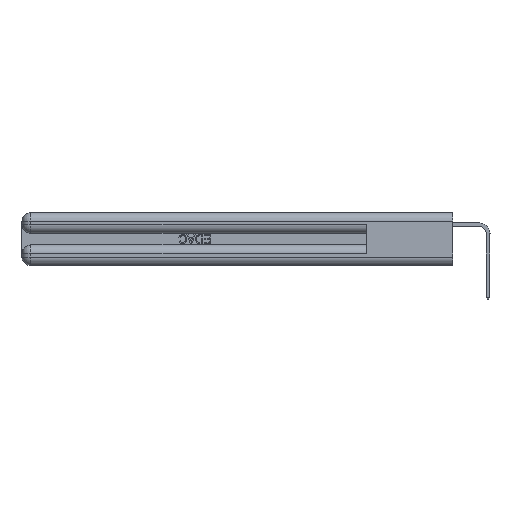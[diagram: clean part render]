
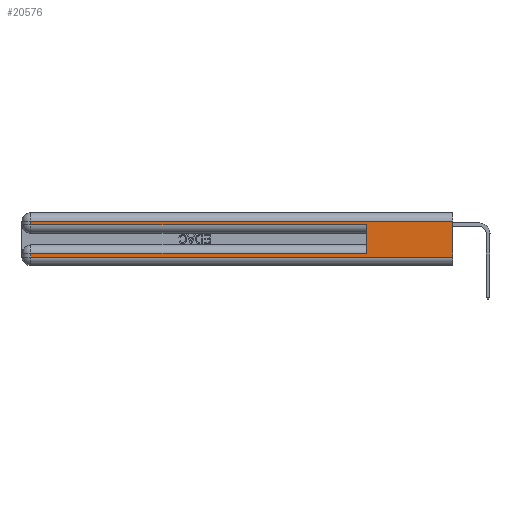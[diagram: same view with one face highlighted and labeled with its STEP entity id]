
A CAD part, left-side view. The second image highlights one B-rep face of the part: STEP entity #20576.
In plain terms, the highlighted planar face has unit normal (-1, 0, 0).
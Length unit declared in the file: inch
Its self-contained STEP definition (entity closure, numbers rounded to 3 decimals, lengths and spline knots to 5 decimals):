
#133 = ORIENTED_EDGE ( 'NONE', *, *, #24252, .T. ) ;
#1194 = DIRECTION ( 'NONE',  ( 0., 0., -1. ) ) ;
#2935 = CARTESIAN_POINT ( 'NONE',  ( 0., 0., 0.06 ) ) ;
#2998 = CARTESIAN_POINT ( 'NONE',  ( 0., 0., 0.37 ) ) ;
#3465 = VERTEX_POINT ( 'NONE', #11335 ) ;
#4004 = CARTESIAN_POINT ( 'NONE',  ( 0., 0.6, 0.085 ) ) ;
#6084 = CARTESIAN_POINT ( 'NONE',  ( 0., 0., 0.37 ) ) ;
#8313 = ORIENTED_EDGE ( 'NONE', *, *, #27761, .T. ) ;
#8512 = VECTOR ( 'NONE', #30366, 39.37008 ) ;
#9287 = VECTOR ( 'NONE', #34190, 39.37008 ) ;
#9555 = VERTEX_POINT ( 'NONE', #49953 ) ;
#9763 = LINE ( 'NONE', #2998, #8512 ) ;
#10040 = DIRECTION ( 'NONE',  ( 0., 0., -1. ) ) ;
#11335 = CARTESIAN_POINT ( 'NONE',  ( 0., 2.94, 0.085 ) ) ;
#12942 = CARTESIAN_POINT ( 'NONE',  ( 0., 2.94, 0.37 ) ) ;
#12971 = ORIENTED_EDGE ( 'NONE', *, *, #31565, .F. ) ;
#13448 = ORIENTED_EDGE ( 'NONE', *, *, #25175, .T. ) ;
#13762 = VECTOR ( 'NONE', #42012, 39.37008 ) ;
#15548 = ORIENTED_EDGE ( 'NONE', *, *, #28218, .T. ) ;
#15988 = VERTEX_POINT ( 'NONE', #4004 ) ;
#17159 = VECTOR ( 'NONE', #33457, 39.37008 ) ;
#17168 = VERTEX_POINT ( 'NONE', #26956 ) ;
#18321 = CARTESIAN_POINT ( 'NONE',  ( 0., 0.6, 0.145 ) ) ;
#20576 = ADVANCED_FACE ( 'NONE', ( #29688 ), #48687, .F. ) ;
#24252 = EDGE_CURVE ( 'NONE', #3465, #46593, #37487, .T. ) ;
#24540 = EDGE_LOOP ( 'NONE', ( #46017, #38470, #13448, #15548, #12971, #46835, #133, #8313 ) ) ;
#24818 = CARTESIAN_POINT ( 'NONE',  ( 0., 0., 0.06 ) ) ;
#24884 = VECTOR ( 'NONE', #47557, 39.37008 ) ;
#25175 = EDGE_CURVE ( 'NONE', #27025, #17168, #44715, .T. ) ;
#25419 = DIRECTION ( 'NONE',  ( 0., 1., 0. ) ) ;
#26956 = CARTESIAN_POINT ( 'NONE',  ( 0., 2.94, 0.285 ) ) ;
#27025 = VERTEX_POINT ( 'NONE', #48936 ) ;
#27183 = VECTOR ( 'NONE', #1194, 39.37008 ) ;
#27510 = LINE ( 'NONE', #44955, #17159 ) ;
#27761 = EDGE_CURVE ( 'NONE', #46593, #43760, #40271, .T. ) ;
#27945 = CARTESIAN_POINT ( 'NONE',  ( 0., 0., 0.085 ) ) ;
#28218 = EDGE_CURVE ( 'NONE', #17168, #9555, #27510, .T. ) ;
#29688 = FACE_OUTER_BOUND ( 'NONE', #24540, .T. ) ;
#30068 = CARTESIAN_POINT ( 'NONE',  ( 0., 2.94, 0.06 ) ) ;
#30366 = DIRECTION ( 'NONE',  ( 0., 0., -1. ) ) ;
#31565 = EDGE_CURVE ( 'NONE', #15988, #9555, #48326, .T. ) ;
#32401 = VERTEX_POINT ( 'NONE', #42156 ) ;
#33327 = AXIS2_PLACEMENT_3D ( 'NONE', #6084, #33336, #10040 ) ;
#33336 = DIRECTION ( 'NONE',  ( 1., 0., 0. ) ) ;
#33457 = DIRECTION ( 'NONE',  ( 0., -1., 0. ) ) ;
#34190 = DIRECTION ( 'NONE',  ( 0., -1., 0. ) ) ;
#35109 = EDGE_CURVE ( 'NONE', #32401, #43760, #9763, .T. ) ;
#36591 = VECTOR ( 'NONE', #25419, 39.37008 ) ;
#37487 = LINE ( 'NONE', #12942, #27183 ) ;
#37796 = LINE ( 'NONE', #44728, #36591 ) ;
#38128 = CARTESIAN_POINT ( 'NONE',  ( 0., 2.94, 0.37 ) ) ;
#38470 = ORIENTED_EDGE ( 'NONE', *, *, #42625, .T. ) ;
#40271 = LINE ( 'NONE', #2935, #9287 ) ;
#41553 = DIRECTION ( 'NONE',  ( 0., 0., 1. ) ) ;
#42012 = DIRECTION ( 'NONE',  ( 0., 0., -1. ) ) ;
#42156 = CARTESIAN_POINT ( 'NONE',  ( 0., 0., 0.31 ) ) ;
#42625 = EDGE_CURVE ( 'NONE', #32401, #27025, #37796, .T. ) ;
#43760 = VERTEX_POINT ( 'NONE', #24818 ) ;
#44715 = LINE ( 'NONE', #38128, #13762 ) ;
#44728 = CARTESIAN_POINT ( 'NONE',  ( 0., 0., 0.31 ) ) ;
#44955 = CARTESIAN_POINT ( 'NONE',  ( 0., 0., 0.285 ) ) ;
#45497 = LINE ( 'NONE', #27945, #24884 ) ;
#46017 = ORIENTED_EDGE ( 'NONE', *, *, #35109, .F. ) ;
#46593 = VERTEX_POINT ( 'NONE', #30068 ) ;
#46835 = ORIENTED_EDGE ( 'NONE', *, *, #50428, .T. ) ;
#47126 = VECTOR ( 'NONE', #41553, 39.37008 ) ;
#47557 = DIRECTION ( 'NONE',  ( 0., 1., 0. ) ) ;
#48326 = LINE ( 'NONE', #18321, #47126 ) ;
#48687 = PLANE ( 'NONE',  #33327 ) ;
#48936 = CARTESIAN_POINT ( 'NONE',  ( 0., 2.94, 0.31 ) ) ;
#49953 = CARTESIAN_POINT ( 'NONE',  ( 0., 0.6, 0.285 ) ) ;
#50428 = EDGE_CURVE ( 'NONE', #15988, #3465, #45497, .T. ) ;
